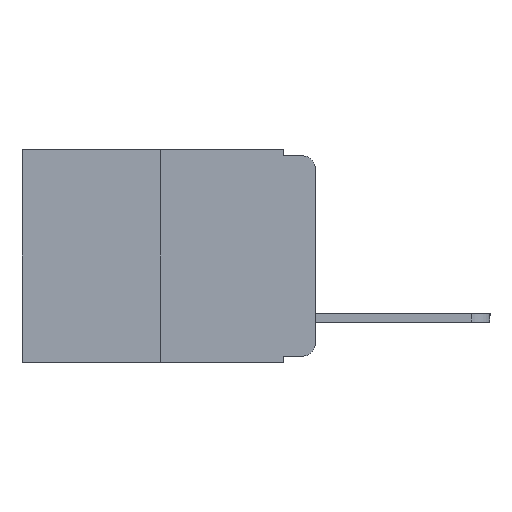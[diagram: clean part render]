
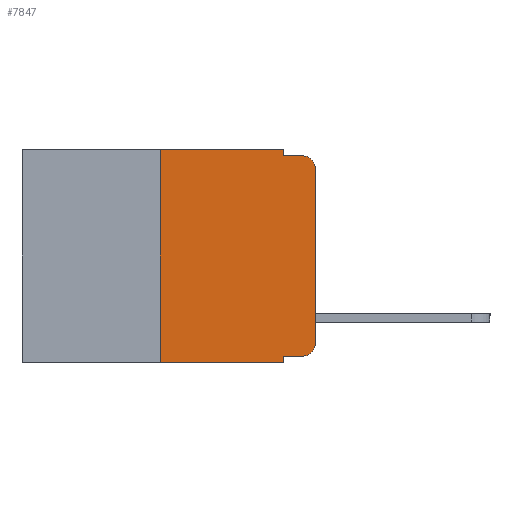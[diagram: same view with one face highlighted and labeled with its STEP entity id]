
A CAD part, left-side view. The second image highlights one B-rep face of the part: STEP entity #7847.
In plain terms, the highlighted planar face has unit normal (-1, 0, 0).
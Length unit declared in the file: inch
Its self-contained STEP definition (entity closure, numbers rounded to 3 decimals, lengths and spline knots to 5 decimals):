
#177 = CARTESIAN_POINT ( 'NONE',  ( 0., 0.25, 0. ) ) ;
#491 = ORIENTED_EDGE ( 'NONE', *, *, #4602, .T. ) ;
#694 = CARTESIAN_POINT ( 'NONE',  ( 0., 0., -0.03 ) ) ;
#1065 = CARTESIAN_POINT ( 'NONE',  ( 0., 0., -0.313 ) ) ;
#1155 = VECTOR ( 'NONE', #9400, 39.37008 ) ;
#1221 = ORIENTED_EDGE ( 'NONE', *, *, #4506, .F. ) ;
#1281 = LINE ( 'NONE', #7657, #1650 ) ;
#1340 = DIRECTION ( 'NONE',  ( 0., 0., -1. ) ) ;
#1359 = CARTESIAN_POINT ( 'NONE',  ( 0., 0.051, 0. ) ) ;
#1409 = DIRECTION ( 'NONE',  ( 0., 0., -1. ) ) ;
#1650 = VECTOR ( 'NONE', #12606, 39.37008 ) ;
#1927 = VERTEX_POINT ( 'NONE', #2308 ) ;
#1984 = AXIS2_PLACEMENT_3D ( 'NONE', #10514, #10296, #10252 ) ;
#2010 = LINE ( 'NONE', #1359, #13042 ) ;
#2145 = ORIENTED_EDGE ( 'NONE', *, *, #4529, .F. ) ;
#2308 = CARTESIAN_POINT ( 'NONE',  ( 0., 0.02, -0.01 ) ) ;
#2689 = ORIENTED_EDGE ( 'NONE', *, *, #4235, .F. ) ;
#3100 = CARTESIAN_POINT ( 'NONE',  ( 0., 0.473, -0.343 ) ) ;
#3190 = LINE ( 'NONE', #3933, #5637 ) ;
#3337 = EDGE_CURVE ( 'NONE', #3735, #9882, #12680, .T. ) ;
#3358 = VERTEX_POINT ( 'NONE', #9477 ) ;
#3499 = ORIENTED_EDGE ( 'NONE', *, *, #11198, .T. ) ;
#3735 = VERTEX_POINT ( 'NONE', #1065 ) ;
#3744 = VECTOR ( 'NONE', #12200, 39.37008 ) ;
#3788 = EDGE_CURVE ( 'NONE', #9882, #1927, #4354, .T. ) ;
#3933 = CARTESIAN_POINT ( 'NONE',  ( 0., 0.25, 0. ) ) ;
#4002 = FACE_OUTER_BOUND ( 'NONE', #8846, .T. ) ;
#4124 = CIRCLE ( 'NONE', #12362, 0.02 ) ;
#4193 = CARTESIAN_POINT ( 'NONE',  ( 0., 0.051, -0.01 ) ) ;
#4235 = EDGE_CURVE ( 'NONE', #8660, #1927, #12240, .T. ) ;
#4324 = EDGE_CURVE ( 'NONE', #11470, #8660, #11097, .T. ) ;
#4354 = CIRCLE ( 'NONE', #1984, 0.02 ) ;
#4506 = EDGE_CURVE ( 'NONE', #10925, #8454, #3190, .T. ) ;
#4529 = EDGE_CURVE ( 'NONE', #3358, #11262, #2010, .T. ) ;
#4549 = EDGE_CURVE ( 'NONE', #3358, #7067, #1281, .T. ) ;
#4602 = EDGE_CURVE ( 'NONE', #7067, #3735, #4124, .T. ) ;
#4739 = ORIENTED_EDGE ( 'NONE', *, *, #3788, .T. ) ;
#4892 = CARTESIAN_POINT ( 'NONE',  ( 0., 0.473, 0. ) ) ;
#5637 = VECTOR ( 'NONE', #13354, 39.37008 ) ;
#5649 = AXIS2_PLACEMENT_3D ( 'NONE', #13139, #8334, #1409 ) ;
#7067 = VERTEX_POINT ( 'NONE', #9187 ) ;
#7226 = ORIENTED_EDGE ( 'NONE', *, *, #4324, .F. ) ;
#7237 = PLANE ( 'NONE',  #5649 ) ;
#7369 = CARTESIAN_POINT ( 'NONE',  ( 0., 0.25, -0.343 ) ) ;
#7551 = ORIENTED_EDGE ( 'NONE', *, *, #3337, .T. ) ;
#7657 = CARTESIAN_POINT ( 'NONE',  ( 0., 0.051, -0.333 ) ) ;
#7847 = ADVANCED_FACE ( 'NONE', ( #4002 ), #7237, .F. ) ;
#8040 = VECTOR ( 'NONE', #11312, 39.37008 ) ;
#8135 = CARTESIAN_POINT ( 'NONE',  ( 0., 0.051, 0. ) ) ;
#8334 = DIRECTION ( 'NONE',  ( 1., 0., 0. ) ) ;
#8454 = VERTEX_POINT ( 'NONE', #177 ) ;
#8660 = VERTEX_POINT ( 'NONE', #4193 ) ;
#8846 = EDGE_LOOP ( 'NONE', ( #7551, #4739, #2689, #7226, #9283, #1221, #3499, #2145, #9322, #491 ) ) ;
#8981 = EDGE_CURVE ( 'NONE', #8454, #11470, #12660, .T. ) ;
#9187 = CARTESIAN_POINT ( 'NONE',  ( 0., 0.02, -0.333 ) ) ;
#9283 = ORIENTED_EDGE ( 'NONE', *, *, #8981, .F. ) ;
#9322 = ORIENTED_EDGE ( 'NONE', *, *, #4549, .T. ) ;
#9400 = DIRECTION ( 'NONE',  ( 0., 0., 1. ) ) ;
#9477 = CARTESIAN_POINT ( 'NONE',  ( 0., 0.051, -0.333 ) ) ;
#9485 = DIRECTION ( 'NONE',  ( 0., 0., -1. ) ) ;
#9519 = CARTESIAN_POINT ( 'NONE',  ( 0., 0.051, 0. ) ) ;
#9882 = VERTEX_POINT ( 'NONE', #694 ) ;
#10166 = CARTESIAN_POINT ( 'NONE',  ( 0., 0.051, -0.01 ) ) ;
#10252 = DIRECTION ( 'NONE',  ( 0., 0., -1. ) ) ;
#10296 = DIRECTION ( 'NONE',  ( -1., 0., 0. ) ) ;
#10514 = CARTESIAN_POINT ( 'NONE',  ( 0., 0.02, -0.03 ) ) ;
#10699 = CARTESIAN_POINT ( 'NONE',  ( 0., 0., 0. ) ) ;
#10801 = CARTESIAN_POINT ( 'NONE',  ( 0., 0.02, -0.313 ) ) ;
#10925 = VERTEX_POINT ( 'NONE', #7369 ) ;
#11097 = LINE ( 'NONE', #9519, #13172 ) ;
#11198 = EDGE_CURVE ( 'NONE', #10925, #11262, #11209, .T. ) ;
#11209 = LINE ( 'NONE', #3100, #13272 ) ;
#11262 = VERTEX_POINT ( 'NONE', #12693 ) ;
#11312 = DIRECTION ( 'NONE',  ( 0., -1., 0. ) ) ;
#11470 = VERTEX_POINT ( 'NONE', #8135 ) ;
#11781 = DIRECTION ( 'NONE',  ( 0., -1., 0. ) ) ;
#12200 = DIRECTION ( 'NONE',  ( 0., -1., 0. ) ) ;
#12240 = LINE ( 'NONE', #10166, #3744 ) ;
#12362 = AXIS2_PLACEMENT_3D ( 'NONE', #10801, #12980, #12894 ) ;
#12606 = DIRECTION ( 'NONE',  ( 0., -1., 0. ) ) ;
#12660 = LINE ( 'NONE', #4892, #8040 ) ;
#12680 = LINE ( 'NONE', #10699, #1155 ) ;
#12693 = CARTESIAN_POINT ( 'NONE',  ( 0., 0.051, -0.343 ) ) ;
#12894 = DIRECTION ( 'NONE',  ( 0., 0., -1. ) ) ;
#12980 = DIRECTION ( 'NONE',  ( -1., 0., 0. ) ) ;
#13042 = VECTOR ( 'NONE', #1340, 39.37008 ) ;
#13139 = CARTESIAN_POINT ( 'NONE',  ( 0., 0.473, 0. ) ) ;
#13172 = VECTOR ( 'NONE', #9485, 39.37008 ) ;
#13272 = VECTOR ( 'NONE', #11781, 39.37008 ) ;
#13354 = DIRECTION ( 'NONE',  ( 0., 0., 1. ) ) ;
